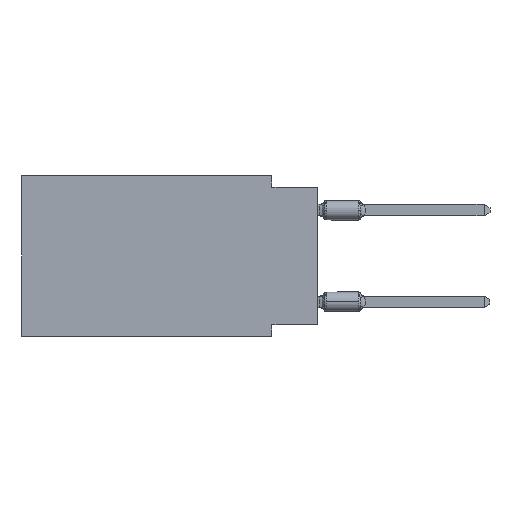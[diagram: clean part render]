
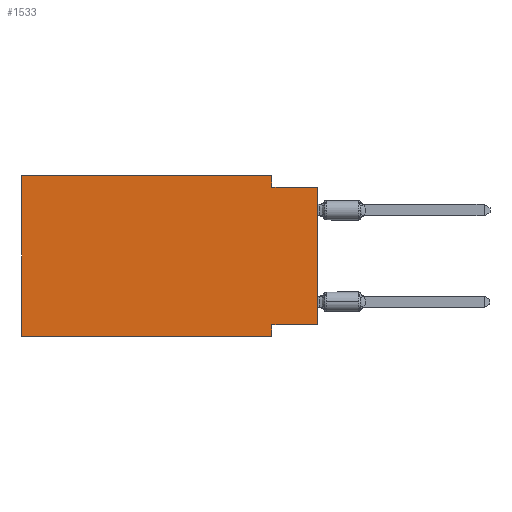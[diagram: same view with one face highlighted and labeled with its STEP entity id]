
A CAD part, left-side view. The second image highlights one B-rep face of the part: STEP entity #1533.
In plain terms, the highlighted planar face has unit normal (-1, 0, 0).
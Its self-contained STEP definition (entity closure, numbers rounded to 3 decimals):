
#134 = CARTESIAN_POINT ( 'NONE',  ( 0., 2.54, 0. ) ) ;
#410 = CARTESIAN_POINT ( 'NONE',  ( 0., 0., -8.255 ) ) ;
#505 = EDGE_CURVE ( 'NONE', #5477, #3064, #4032, .T. ) ;
#684 = VERTEX_POINT ( 'NONE', #410 ) ;
#803 = DIRECTION ( 'NONE',  ( 0., -1., 0. ) ) ;
#971 = CARTESIAN_POINT ( 'NONE',  ( 0., 2.54, -0.635 ) ) ;
#1533 = ADVANCED_FACE ( 'NONE', ( #12311 ), #17969, .F. ) ;
#1910 = AXIS2_PLACEMENT_3D ( 'NONE', #5242, #18064, #10911 ) ;
#2441 = DIRECTION ( 'NONE',  ( 0., -1., 0. ) ) ;
#2476 = CARTESIAN_POINT ( 'NONE',  ( 0., 2.54, -8.89 ) ) ;
#2508 = CARTESIAN_POINT ( 'NONE',  ( 0., 0., -0.635 ) ) ;
#2650 = VECTOR ( 'NONE', #2441, 1000. ) ;
#3064 = VERTEX_POINT ( 'NONE', #971 ) ;
#3070 = VERTEX_POINT ( 'NONE', #16384 ) ;
#3189 = LINE ( 'NONE', #7479, #8585 ) ;
#3428 = VECTOR ( 'NONE', #5696, 1000. ) ;
#3455 = EDGE_CURVE ( 'NONE', #3070, #8908, #9166, .T. ) ;
#3915 = CARTESIAN_POINT ( 'NONE',  ( 0., 0., -0.635 ) ) ;
#4032 = LINE ( 'NONE', #134, #6921 ) ;
#5231 = EDGE_CURVE ( 'NONE', #684, #13070, #5504, .T. ) ;
#5242 = CARTESIAN_POINT ( 'NONE',  ( 0., 16.383, 0. ) ) ;
#5477 = VERTEX_POINT ( 'NONE', #9127 ) ;
#5504 = LINE ( 'NONE', #6910, #3428 ) ;
#5696 = DIRECTION ( 'NONE',  ( 0., 0., 1. ) ) ;
#5975 = ORIENTED_EDGE ( 'NONE', *, *, #16861, .F. ) ;
#5983 = CARTESIAN_POINT ( 'NONE',  ( 0., 16.383, 0. ) ) ;
#6910 = CARTESIAN_POINT ( 'NONE',  ( 0., 0., 0. ) ) ;
#6921 = VECTOR ( 'NONE', #16855, 1000. ) ;
#7341 = VECTOR ( 'NONE', #803, 1000. ) ;
#7479 = CARTESIAN_POINT ( 'NONE',  ( 0., 16.383, 0. ) ) ;
#7983 = VECTOR ( 'NONE', #14447, 1000. ) ;
#8142 = DIRECTION ( 'NONE',  ( 0., 0., -1. ) ) ;
#8376 = ORIENTED_EDGE ( 'NONE', *, *, #9045, .F. ) ;
#8585 = VECTOR ( 'NONE', #15918, 1000. ) ;
#8833 = ORIENTED_EDGE ( 'NONE', *, *, #11306, .F. ) ;
#8908 = VERTEX_POINT ( 'NONE', #12531 ) ;
#9045 = EDGE_CURVE ( 'NONE', #684, #18217, #13173, .T. ) ;
#9127 = CARTESIAN_POINT ( 'NONE',  ( 0., 2.54, 0. ) ) ;
#9166 = LINE ( 'NONE', #13713, #7341 ) ;
#9331 = EDGE_CURVE ( 'NONE', #18217, #8908, #16774, .T. ) ;
#9365 = CARTESIAN_POINT ( 'NONE',  ( 0., 16.383, 0. ) ) ;
#9661 = ORIENTED_EDGE ( 'NONE', *, *, #505, .F. ) ;
#10808 = CARTESIAN_POINT ( 'NONE',  ( 0., 2.54, -8.255 ) ) ;
#10911 = DIRECTION ( 'NONE',  ( 0., 0., -1. ) ) ;
#11227 = ORIENTED_EDGE ( 'NONE', *, *, #5231, .T. ) ;
#11306 = EDGE_CURVE ( 'NONE', #14944, #5477, #3189, .T. ) ;
#11493 = EDGE_CURVE ( 'NONE', #3064, #13070, #14138, .T. ) ;
#11510 = ORIENTED_EDGE ( 'NONE', *, *, #9331, .F. ) ;
#12311 = FACE_OUTER_BOUND ( 'NONE', #13137, .T. ) ;
#12531 = CARTESIAN_POINT ( 'NONE',  ( 0., 2.54, -8.89 ) ) ;
#12810 = VECTOR ( 'NONE', #17346, 1000. ) ;
#13070 = VERTEX_POINT ( 'NONE', #2508 ) ;
#13137 = EDGE_LOOP ( 'NONE', ( #11227, #16452, #9661, #8833, #5975, #15012, #11510, #8376 ) ) ;
#13173 = LINE ( 'NONE', #15678, #12810 ) ;
#13713 = CARTESIAN_POINT ( 'NONE',  ( 0., 16.383, -8.89 ) ) ;
#14138 = LINE ( 'NONE', #3915, #2650 ) ;
#14447 = DIRECTION ( 'NONE',  ( 0., 0., 1. ) ) ;
#14547 = LINE ( 'NONE', #5983, #7983 ) ;
#14944 = VERTEX_POINT ( 'NONE', #9365 ) ;
#15012 = ORIENTED_EDGE ( 'NONE', *, *, #3455, .T. ) ;
#15678 = CARTESIAN_POINT ( 'NONE',  ( 0., 0., -8.255 ) ) ;
#15759 = VECTOR ( 'NONE', #8142, 1000. ) ;
#15918 = DIRECTION ( 'NONE',  ( 0., -1., 0. ) ) ;
#16384 = CARTESIAN_POINT ( 'NONE',  ( 0., 16.383, -8.89 ) ) ;
#16452 = ORIENTED_EDGE ( 'NONE', *, *, #11493, .F. ) ;
#16774 = LINE ( 'NONE', #2476, #15759 ) ;
#16855 = DIRECTION ( 'NONE',  ( 0., 0., -1. ) ) ;
#16861 = EDGE_CURVE ( 'NONE', #3070, #14944, #14547, .T. ) ;
#17346 = DIRECTION ( 'NONE',  ( 0., 1., 0. ) ) ;
#17969 = PLANE ( 'NONE',  #1910 ) ;
#18064 = DIRECTION ( 'NONE',  ( 1., 0., 0. ) ) ;
#18217 = VERTEX_POINT ( 'NONE', #10808 ) ;
